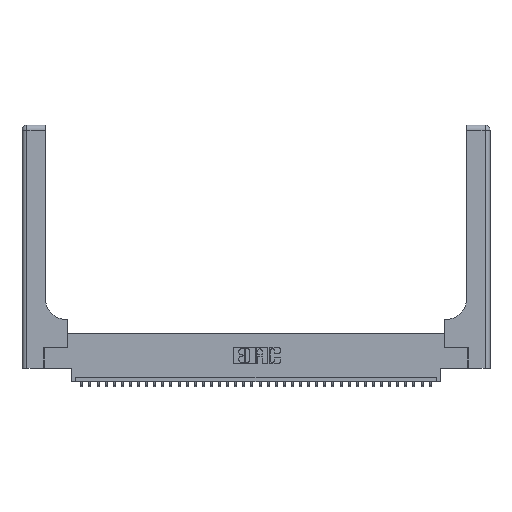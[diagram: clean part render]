
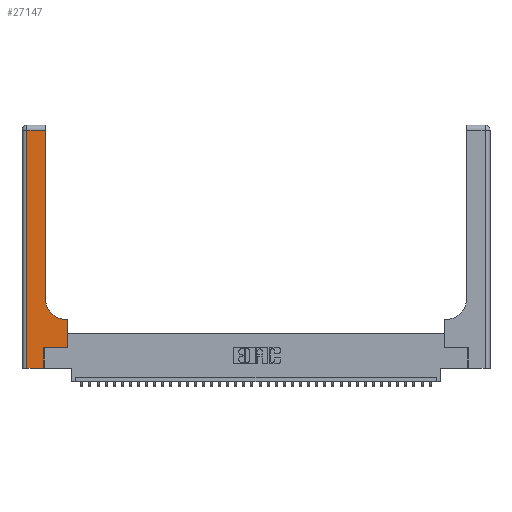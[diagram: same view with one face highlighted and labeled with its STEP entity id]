
A CAD part, top view. The second image highlights one B-rep face of the part: STEP entity #27147.
In plain terms, the highlighted planar face has unit normal (0, 0, 1).
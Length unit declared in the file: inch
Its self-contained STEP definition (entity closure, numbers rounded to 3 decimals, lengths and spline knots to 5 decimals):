
#67 = VECTOR ( 'NONE', #25180, 39.37008 ) ;
#816 = EDGE_CURVE ( 'NONE', #12449, #17395, #7990, .T. ) ;
#1031 = VECTOR ( 'NONE', #21992, 39.37008 ) ;
#1589 = DIRECTION ( 'NONE',  ( 1., 0., 0. ) ) ;
#1788 = DIRECTION ( 'NONE',  ( 0., 1., 0. ) ) ;
#2104 = CARTESIAN_POINT ( 'NONE',  ( 0.269, 0., 0.37 ) ) ;
#3329 = EDGE_CURVE ( 'NONE', #14626, #36703, #5699, .T. ) ;
#3572 = EDGE_CURVE ( 'NONE', #28022, #14626, #26938, .T. ) ;
#3590 = PLANE ( 'NONE',  #31750 ) ;
#4377 = CARTESIAN_POINT ( 'NONE',  ( 0.06, 0., 0.37 ) ) ;
#5027 = VERTEX_POINT ( 'NONE', #9235 ) ;
#5233 = VECTOR ( 'NONE', #23075, 39.37008 ) ;
#5699 = LINE ( 'NONE', #23198, #5233 ) ;
#5784 = EDGE_CURVE ( 'NONE', #36703, #12449, #38188, .T. ) ;
#6531 = VECTOR ( 'NONE', #30126, 39.37008 ) ;
#7191 = CARTESIAN_POINT ( 'NONE',  ( 0.06, 3., 0.37 ) ) ;
#7979 = CARTESIAN_POINT ( 'NONE',  ( 0.269, 0.25, 0.37 ) ) ;
#7990 = LINE ( 'NONE', #22613, #31230 ) ;
#9060 = DIRECTION ( 'NONE',  ( 1., 0., 0. ) ) ;
#9144 = CARTESIAN_POINT ( 'NONE',  ( 0.5415, 0.85, 0.37 ) ) ;
#9235 = CARTESIAN_POINT ( 'NONE',  ( 0.269, 0.25, 0.37 ) ) ;
#9883 = FACE_OUTER_BOUND ( 'NONE', #35304, .T. ) ;
#10131 = ORIENTED_EDGE ( 'NONE', *, *, #13585, .T. ) ;
#10367 = ORIENTED_EDGE ( 'NONE', *, *, #17189, .T. ) ;
#10385 = CARTESIAN_POINT ( 'NONE',  ( 0.269, 0., 0.37 ) ) ;
#10916 = CARTESIAN_POINT ( 'NONE',  ( 0.06, 2.94, 0.37 ) ) ;
#12167 = DIRECTION ( 'NONE',  ( 1., 0., 0. ) ) ;
#12449 = VERTEX_POINT ( 'NONE', #31030 ) ;
#12936 = DIRECTION ( 'NONE',  ( -1., 0., 0. ) ) ;
#12938 = CARTESIAN_POINT ( 'NONE',  ( 0.5585, 0.25, 0.37 ) ) ;
#13033 = LINE ( 'NONE', #13551, #67 ) ;
#13525 = EDGE_CURVE ( 'NONE', #27745, #5027, #21373, .T. ) ;
#13551 = CARTESIAN_POINT ( 'NONE',  ( 0., 2.94, 0.37 ) ) ;
#13585 = EDGE_CURVE ( 'NONE', #23352, #37203, #32077, .T. ) ;
#14308 = EDGE_CURVE ( 'NONE', #17395, #23352, #13033, .T. ) ;
#14529 = DIRECTION ( 'NONE',  ( 0., 1., 0. ) ) ;
#14579 = VECTOR ( 'NONE', #1589, 39.37008 ) ;
#14626 = VERTEX_POINT ( 'NONE', #31777 ) ;
#17189 = EDGE_CURVE ( 'NONE', #37203, #27745, #31310, .T. ) ;
#17395 = VERTEX_POINT ( 'NONE', #28464 ) ;
#17670 = VECTOR ( 'NONE', #14529, 39.37008 ) ;
#20930 = ORIENTED_EDGE ( 'NONE', *, *, #816, .T. ) ;
#21171 = DIRECTION ( 'NONE',  ( 0., 0., -1. ) ) ;
#21373 = LINE ( 'NONE', #10385, #17670 ) ;
#21992 = DIRECTION ( 'NONE',  ( 0., -1., 0. ) ) ;
#22172 = ORIENTED_EDGE ( 'NONE', *, *, #3329, .T. ) ;
#22613 = CARTESIAN_POINT ( 'NONE',  ( 0.2915, 3., 0.37 ) ) ;
#22912 = CARTESIAN_POINT ( 'NONE',  ( 0.5415, 0.6, 0.37 ) ) ;
#23075 = DIRECTION ( 'NONE',  ( -1., 0., 0. ) ) ;
#23198 = CARTESIAN_POINT ( 'NONE',  ( 0.2915, 0.6, 0.37 ) ) ;
#23352 = VERTEX_POINT ( 'NONE', #10916 ) ;
#23572 = AXIS2_PLACEMENT_3D ( 'NONE', #9144, #29859, #12167 ) ;
#23793 = ORIENTED_EDGE ( 'NONE', *, *, #34285, .T. ) ;
#24419 = ORIENTED_EDGE ( 'NONE', *, *, #14308, .T. ) ;
#24749 = ORIENTED_EDGE ( 'NONE', *, *, #3572, .T. ) ;
#25180 = DIRECTION ( 'NONE',  ( -1., 0., 0. ) ) ;
#26118 = CARTESIAN_POINT ( 'NONE',  ( 0., 0., 0.37 ) ) ;
#26938 = LINE ( 'NONE', #33243, #6531 ) ;
#27147 = ADVANCED_FACE ( 'NONE', ( #9883 ), #3590, .F. ) ;
#27745 = VERTEX_POINT ( 'NONE', #2104 ) ;
#28022 = VERTEX_POINT ( 'NONE', #12938 ) ;
#28078 = ORIENTED_EDGE ( 'NONE', *, *, #13525, .T. ) ;
#28464 = CARTESIAN_POINT ( 'NONE',  ( 0.2915, 2.94, 0.37 ) ) ;
#29859 = DIRECTION ( 'NONE',  ( 0., 0., -1. ) ) ;
#30126 = DIRECTION ( 'NONE',  ( 0., 1., 0. ) ) ;
#30629 = CARTESIAN_POINT ( 'NONE',  ( 0., 3., 0.37 ) ) ;
#31030 = CARTESIAN_POINT ( 'NONE',  ( 0.2915, 0.85, 0.37 ) ) ;
#31230 = VECTOR ( 'NONE', #1788, 39.37008 ) ;
#31310 = LINE ( 'NONE', #26118, #37259 ) ;
#31629 = ORIENTED_EDGE ( 'NONE', *, *, #5784, .T. ) ;
#31750 = AXIS2_PLACEMENT_3D ( 'NONE', #30629, #21171, #12936 ) ;
#31777 = CARTESIAN_POINT ( 'NONE',  ( 0.5585, 0.6, 0.37 ) ) ;
#32077 = LINE ( 'NONE', #7191, #1031 ) ;
#33243 = CARTESIAN_POINT ( 'NONE',  ( 0.5585, 0.25, 0.37 ) ) ;
#34285 = EDGE_CURVE ( 'NONE', #5027, #28022, #37626, .T. ) ;
#35304 = EDGE_LOOP ( 'NONE', ( #20930, #24419, #10131, #10367, #28078, #23793, #24749, #22172, #31629 ) ) ;
#36703 = VERTEX_POINT ( 'NONE', #22912 ) ;
#37203 = VERTEX_POINT ( 'NONE', #4377 ) ;
#37259 = VECTOR ( 'NONE', #9060, 39.37008 ) ;
#37626 = LINE ( 'NONE', #7979, #14579 ) ;
#38188 = CIRCLE ( 'NONE', #23572, 0.25 ) ;
